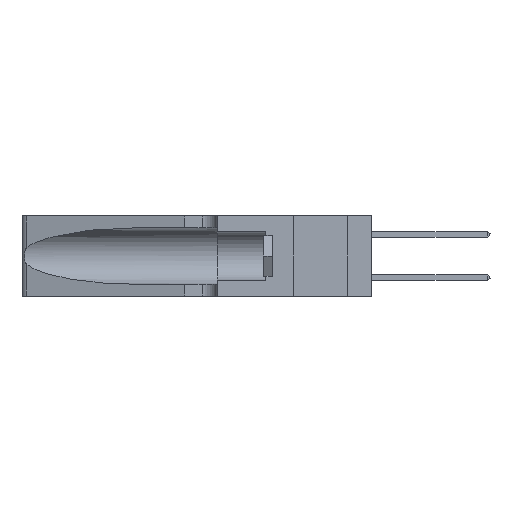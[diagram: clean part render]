
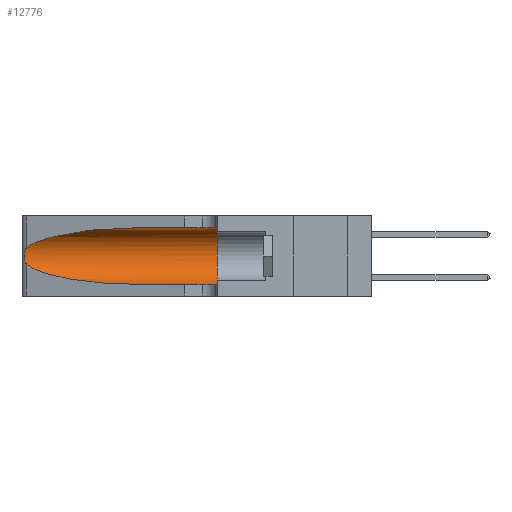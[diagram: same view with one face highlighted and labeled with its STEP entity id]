
A CAD part, left-side view. The second image highlights one B-rep face of the part: STEP entity #12776.
In plain terms, the highlighted cylindrical face has radius 3.308 mm (diameter 6.617 mm), a partial arc.
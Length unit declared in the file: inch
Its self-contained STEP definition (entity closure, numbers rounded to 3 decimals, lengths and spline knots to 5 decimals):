
#167 = CARTESIAN_POINT ( 'NONE',  ( 0.25639, 1.23184, 0.21858 ) ) ;
#1152 = EDGE_CURVE ( 'NONE', #11893, #12999, #23066, .T. ) ;
#1676 = AXIS2_PLACEMENT_3D ( 'NONE', #2945, #19153, #25348 ) ;
#1761 = CYLINDRICAL_SURFACE ( 'NONE', #22373, 0.13025 ) ;
#2069 = LINE ( 'NONE', #25206, #16941 ) ;
#2259 = CARTESIAN_POINT ( 'NONE',  ( 0.26075, 1.23896, 0.19203 ) ) ;
#2288 =( BOUNDED_CURVE ( )  B_SPLINE_CURVE ( 3, ( #24477, #10281, #22455, #14202 ),
 .UNSPECIFIED., .F., .F. ) 
 B_SPLINE_CURVE_WITH_KNOTS ( ( 4, 4 ),
 ( 3.44316, 4.71239 ),
 .UNSPECIFIED. ) 
 CURVE ( )  GEOMETRIC_REPRESENTATION_ITEM ( )  RATIONAL_B_SPLINE_CURVE ( ( 1., 0.87, 0.87, 1. ) ) 
 REPRESENTATION_ITEM ( '' )  );
#2678 = EDGE_CURVE ( 'NONE', #25211, #11019, #7530, .T. ) ;
#2945 = CARTESIAN_POINT ( 'NONE',  ( 0.1305, 0.35, 0.185 ) ) ;
#3074 = DIRECTION ( 'NONE',  ( 0., -1., 0. ) ) ;
#3188 = EDGE_LOOP ( 'NONE', ( #21549, #23172, #9289, #23987, #15773, #9479 ) ) ;
#3484 = CARTESIAN_POINT ( 'NONE',  ( 0.25487, 1.22718, 0.22369 ) ) ;
#4101 = CARTESIAN_POINT ( 'NONE',  ( 0.25555, 1.22993, 0.14849 ) ) ;
#4320 = CARTESIAN_POINT ( 'NONE',  ( 0.26017, 1.23833, 0.17102 ) ) ;
#5793 = EDGE_CURVE ( 'NONE', #12999, #15660, #23546, .T. ) ;
#6083 = CARTESIAN_POINT ( 'NONE',  ( 0.26075, 1.23896, 0.178 ) ) ;
#6608 = CARTESIAN_POINT ( 'NONE',  ( 0.25856, 1.23593, 0.16098 ) ) ;
#7237 = CARTESIAN_POINT ( 'NONE',  ( 0.1305, 0.35, 0.05475 ) ) ;
#7422 = DIRECTION ( 'NONE',  ( 0., -1., 0. ) ) ;
#7530 = CIRCLE ( 'NONE', #1676, 0.13025 ) ;
#7805 = EDGE_CURVE ( 'NONE', #15660, #13323, #2288, .T. ) ;
#7988 = VECTOR ( 'NONE', #8696, 39.37008 ) ;
#8439 = CARTESIAN_POINT ( 'NONE',  ( 0.25854, 1.2359, 0.20912 ) ) ;
#8508 = CARTESIAN_POINT ( 'NONE',  ( 0.1305, 0.72297, 0.31525 ) ) ;
#8696 = DIRECTION ( 'NONE',  ( 0., -1., 0. ) ) ;
#9289 = ORIENTED_EDGE ( 'NONE', *, *, #7805, .T. ) ;
#9479 = ORIENTED_EDGE ( 'NONE', *, *, #24700, .F. ) ;
#10281 = CARTESIAN_POINT ( 'NONE',  ( 0.2373, 1.15595, 0.08982 ) ) ;
#11019 = VERTEX_POINT ( 'NONE', #7237 ) ;
#11401 = EDGE_CURVE ( 'NONE', #13323, #11019, #14040, .T. ) ;
#11893 = VERTEX_POINT ( 'NONE', #8508 ) ;
#12347 = CARTESIAN_POINT ( 'NONE',  ( 0.25487, 1.22718, 0.14631 ) ) ;
#12620 = CARTESIAN_POINT ( 'NONE',  ( 0.2373, 1.15595, 0.28018 ) ) ;
#12776 = ADVANCED_FACE ( 'NONE', ( #25499 ), #1761, .F. ) ;
#12999 = VERTEX_POINT ( 'NONE', #20010 ) ;
#13267 = CARTESIAN_POINT ( 'NONE',  ( 0.1305, 0.72297, 0.05475 ) ) ;
#13323 = VERTEX_POINT ( 'NONE', #13267 ) ;
#14040 = LINE ( 'NONE', #22821, #7988 ) ;
#14202 = CARTESIAN_POINT ( 'NONE',  ( 0.1305, 0.72297, 0.05475 ) ) ;
#15660 = VERTEX_POINT ( 'NONE', #20606 ) ;
#15773 = ORIENTED_EDGE ( 'NONE', *, *, #2678, .F. ) ;
#16419 = CARTESIAN_POINT ( 'NONE',  ( 0.25639, 1.23186, 0.15144 ) ) ;
#16874 = CARTESIAN_POINT ( 'NONE',  ( 0.25555, 1.22994, 0.2215 ) ) ;
#16941 = VECTOR ( 'NONE', #3074, 39.37008 ) ;
#18644 = CARTESIAN_POINT ( 'NONE',  ( 0.25789, 1.23486, 0.15765 ) ) ;
#19153 = DIRECTION ( 'NONE',  ( 0., 1., 0. ) ) ;
#19837 = CARTESIAN_POINT ( 'NONE',  ( 0.1305, 1.61858, 0.185 ) ) ;
#20010 = CARTESIAN_POINT ( 'NONE',  ( 0.25487, 1.22718, 0.22369 ) ) ;
#20322 = CARTESIAN_POINT ( 'NONE',  ( 0.1305, 0.35, 0.31525 ) ) ;
#20606 = CARTESIAN_POINT ( 'NONE',  ( 0.25487, 1.22718, 0.14631 ) ) ;
#21549 = ORIENTED_EDGE ( 'NONE', *, *, #1152, .T. ) ;
#21575 = CARTESIAN_POINT ( 'NONE',  ( 0.25787, 1.23484, 0.2124 ) ) ;
#21899 = DIRECTION ( 'NONE',  ( 0., 0., -1. ) ) ;
#22373 = AXIS2_PLACEMENT_3D ( 'NONE', #19837, #7422, #21899 ) ;
#22455 = CARTESIAN_POINT ( 'NONE',  ( 0.18966, 0.96281, 0.05475 ) ) ;
#22821 = CARTESIAN_POINT ( 'NONE',  ( 0.1305, 1.61858, 0.05475 ) ) ;
#22890 = CARTESIAN_POINT ( 'NONE',  ( 0.1305, 0.72297, 0.31525 ) ) ;
#23066 =( BOUNDED_CURVE ( )  B_SPLINE_CURVE ( 3, ( #22890, #23072, #12620, #24664 ),
 .UNSPECIFIED., .F., .T. ) 
 B_SPLINE_CURVE_WITH_KNOTS ( ( 4, 4 ),
 ( 1.5708, 2.84003 ),
 .UNSPECIFIED. ) 
 CURVE ( )  GEOMETRIC_REPRESENTATION_ITEM ( )  RATIONAL_B_SPLINE_CURVE ( ( 1., 0.87, 0.87, 1. ) ) 
 REPRESENTATION_ITEM ( '' )  );
#23072 = CARTESIAN_POINT ( 'NONE',  ( 0.18966, 0.96281, 0.31525 ) ) ;
#23172 = ORIENTED_EDGE ( 'NONE', *, *, #5793, .T. ) ;
#23546 = B_SPLINE_CURVE_WITH_KNOTS ( 'NONE', 3,
 ( #3484, #16874, #167, #21575, #8439, #23570, #2259, #6083, #4320, #6608, #18644, #16419, #4101, #12347 ),
 .UNSPECIFIED., .F., .F.,
 ( 4, 2, 2, 2, 2, 2, 4 ),
 ( 0., 0.00027, 0.00053, 0.00107, 0.0016, 0.00187, 0.00214 ),
 .UNSPECIFIED. ) ;
#23570 = CARTESIAN_POINT ( 'NONE',  ( 0.26018, 1.23835, 0.19895 ) ) ;
#23987 = ORIENTED_EDGE ( 'NONE', *, *, #11401, .T. ) ;
#24477 = CARTESIAN_POINT ( 'NONE',  ( 0.25487, 1.22718, 0.14631 ) ) ;
#24664 = CARTESIAN_POINT ( 'NONE',  ( 0.25487, 1.22718, 0.22369 ) ) ;
#24700 = EDGE_CURVE ( 'NONE', #11893, #25211, #2069, .T. ) ;
#25206 = CARTESIAN_POINT ( 'NONE',  ( 0.1305, 1.61858, 0.31525 ) ) ;
#25211 = VERTEX_POINT ( 'NONE', #20322 ) ;
#25348 = DIRECTION ( 'NONE',  ( 0., 0., 1. ) ) ;
#25499 = FACE_OUTER_BOUND ( 'NONE', #3188, .T. ) ;
